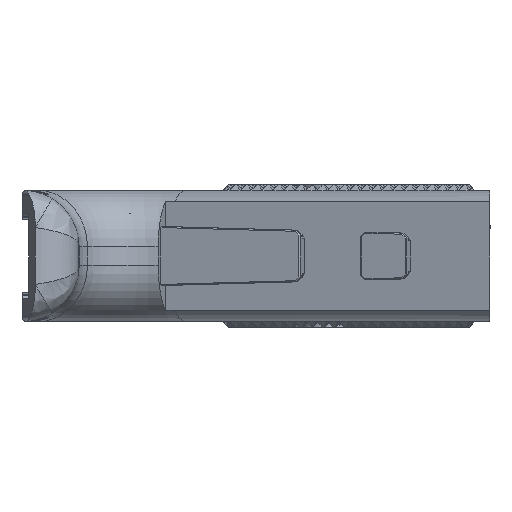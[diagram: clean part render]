
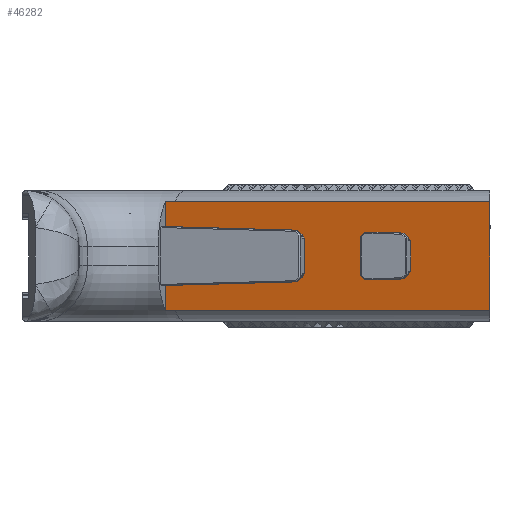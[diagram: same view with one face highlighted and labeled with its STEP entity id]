
A CAD part, left-side view. The second image highlights one B-rep face of the part: STEP entity #46282.
In plain terms, the highlighted planar face has unit normal (-0.951, 0.309, 0).
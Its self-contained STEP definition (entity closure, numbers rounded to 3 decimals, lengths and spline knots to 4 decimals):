
#57=FACE_BOUND('',#19786,.T.);
#5211=LINE('',#88973,#10780);
#5229=LINE('',#89011,#10798);
#5237=LINE('',#89028,#10806);
#5242=LINE('',#89037,#10811);
#5244=LINE('',#89040,#10813);
#5246=LINE('',#89045,#10815);
#5248=LINE('',#89049,#10817);
#5250=LINE('',#89052,#10819);
#5252=LINE('',#89056,#10821);
#5253=LINE('',#89058,#10822);
#5259=LINE('',#89071,#10828);
#5261=LINE('',#89075,#10830);
#5262=LINE('',#89078,#10831);
#5264=LINE('',#89082,#10833);
#5265=LINE('',#89092,#10834);
#5266=LINE('',#89094,#10835);
#5267=LINE('',#89096,#10836);
#5268=LINE('',#89106,#10837);
#5269=LINE('',#89107,#10838);
#10780=VECTOR('',#59780,0.3937);
#10798=VECTOR('',#59816,0.3937);
#10806=VECTOR('',#59830,0.3937);
#10811=VECTOR('',#59839,0.3937);
#10813=VECTOR('',#59843,0.3937);
#10815=VECTOR('',#59847,0.3937);
#10817=VECTOR('',#59851,0.3937);
#10819=VECTOR('',#59855,0.3937);
#10821=VECTOR('',#59859,0.3937);
#10822=VECTOR('',#59862,0.3937);
#10828=VECTOR('',#59878,0.3937);
#10830=VECTOR('',#59882,0.3937);
#10831=VECTOR('',#59885,0.3937);
#10833=VECTOR('',#59889,0.3937);
#10834=VECTOR('',#59890,0.3937);
#10835=VECTOR('',#59891,0.3937);
#10836=VECTOR('',#59892,0.3937);
#10837=VECTOR('',#59893,0.3937);
#10838=VECTOR('',#59894,0.3937);
#13953=PLANE('',#49273);
#16778=FACE_OUTER_BOUND('',#19785,.T.);
#19785=EDGE_LOOP('',(#41315,#41316,#41317,#41318,#41319,#41320,#41321,#41322,
#41323,#41324,#41325,#41326));
#19786=EDGE_LOOP('',(#41327,#41328,#41329,#41330,#41331,#41332,#41333,#41334,
#41335));
#20582=B_SPLINE_CURVE_WITH_KNOTS('',3,(#89084,#89085,#89086,#89087,#89088,
#89089,#89090),.UNSPECIFIED.,.F.,.F.,(4,3,4),(0.,0.1181,0.2155),
 .UNSPECIFIED.);
#20583=B_SPLINE_CURVE_WITH_KNOTS('',3,(#89098,#89099,#89100,#89101,#89102,
#89103,#89104),.UNSPECIFIED.,.F.,.F.,(4,3,4),(-0.2155,-0.1181,
0.),.UNSPECIFIED.);
#23615=VERTEX_POINT('',#88970);
#23616=VERTEX_POINT('',#88972);
#23626=VERTEX_POINT('',#89008);
#23627=VERTEX_POINT('',#89010);
#23632=VERTEX_POINT('',#89025);
#23633=VERTEX_POINT('',#89027);
#23635=VERTEX_POINT('',#89036);
#23636=VERTEX_POINT('',#89042);
#23637=VERTEX_POINT('',#89044);
#23638=VERTEX_POINT('',#89048);
#23639=VERTEX_POINT('',#89054);
#23641=VERTEX_POINT('',#89069);
#23642=VERTEX_POINT('',#89073);
#23643=VERTEX_POINT('',#89077);
#23644=VERTEX_POINT('',#89081);
#23645=VERTEX_POINT('',#89083);
#23646=VERTEX_POINT('',#89091);
#23647=VERTEX_POINT('',#89093);
#23648=VERTEX_POINT('',#89095);
#23649=VERTEX_POINT('',#89097);
#23650=VERTEX_POINT('',#89105);
#29614=EDGE_CURVE('',#23616,#23615,#5211,.T.);
#29632=EDGE_CURVE('',#23626,#23627,#5229,.T.);
#29640=EDGE_CURVE('',#23632,#23633,#5237,.F.);
#29645=EDGE_CURVE('',#23616,#23635,#5242,.F.);
#29647=EDGE_CURVE('',#23632,#23635,#5244,.T.);
#29649=EDGE_CURVE('',#23636,#23637,#5246,.F.);
#29651=EDGE_CURVE('',#23638,#23637,#5248,.T.);
#29653=EDGE_CURVE('',#23636,#23633,#5250,.T.);
#29655=EDGE_CURVE('',#23639,#23615,#5252,.F.);
#29656=EDGE_CURVE('',#23638,#23639,#5253,.F.);
#29662=EDGE_CURVE('',#23641,#23626,#5259,.F.);
#29664=EDGE_CURVE('',#23641,#23642,#5261,.T.);
#29665=EDGE_CURVE('',#23627,#23643,#5262,.F.);
#29667=EDGE_CURVE('',#23644,#23642,#5264,.T.);
#29668=EDGE_CURVE('',#23645,#23644,#20582,.T.);
#29669=EDGE_CURVE('',#23646,#23645,#5265,.T.);
#29670=EDGE_CURVE('',#23647,#23646,#5266,.T.);
#29671=EDGE_CURVE('',#23648,#23647,#5267,.T.);
#29672=EDGE_CURVE('',#23649,#23648,#20583,.T.);
#29673=EDGE_CURVE('',#23650,#23649,#5268,.T.);
#29674=EDGE_CURVE('',#23650,#23643,#5269,.T.);
#41315=ORIENTED_EDGE('',*,*,#29664,.T.);
#41316=ORIENTED_EDGE('',*,*,#29667,.F.);
#41317=ORIENTED_EDGE('',*,*,#29668,.F.);
#41318=ORIENTED_EDGE('',*,*,#29669,.F.);
#41319=ORIENTED_EDGE('',*,*,#29670,.F.);
#41320=ORIENTED_EDGE('',*,*,#29671,.F.);
#41321=ORIENTED_EDGE('',*,*,#29672,.F.);
#41322=ORIENTED_EDGE('',*,*,#29673,.F.);
#41323=ORIENTED_EDGE('',*,*,#29674,.T.);
#41324=ORIENTED_EDGE('',*,*,#29665,.F.);
#41325=ORIENTED_EDGE('',*,*,#29632,.F.);
#41326=ORIENTED_EDGE('',*,*,#29662,.F.);
#41327=ORIENTED_EDGE('',*,*,#29614,.T.);
#41328=ORIENTED_EDGE('',*,*,#29655,.F.);
#41329=ORIENTED_EDGE('',*,*,#29656,.F.);
#41330=ORIENTED_EDGE('',*,*,#29651,.T.);
#41331=ORIENTED_EDGE('',*,*,#29649,.F.);
#41332=ORIENTED_EDGE('',*,*,#29653,.T.);
#41333=ORIENTED_EDGE('',*,*,#29640,.F.);
#41334=ORIENTED_EDGE('',*,*,#29647,.T.);
#41335=ORIENTED_EDGE('',*,*,#29645,.F.);
#46282=ADVANCED_FACE('',(#16778,#57),#13953,.T.);
#49273=AXIS2_PLACEMENT_3D('',#89080,#59887,#59888);
#59780=DIRECTION('',(0.,0.,1.));
#59816=DIRECTION('',(0.,0.,1.));
#59830=DIRECTION('',(0.216,0.664,-0.716));
#59839=DIRECTION('',(0.221,0.681,0.698));
#59843=DIRECTION('',(0.309,0.951,-0.026));
#59847=DIRECTION('',(-0.216,-0.664,-0.716));
#59851=DIRECTION('',(-0.309,-0.951,-0.026));
#59855=DIRECTION('',(0.,0.,-1.));
#59859=DIRECTION('',(-0.12,-0.37,0.921));
#59862=DIRECTION('',(-0.221,-0.681,0.698));
#59878=DIRECTION('',(0.216,0.664,-0.716));
#59882=DIRECTION('',(0.309,0.951,-0.026));
#59885=DIRECTION('',(-0.216,-0.664,-0.716));
#59887=DIRECTION('center_axis',(-0.951,0.309,0.));
#59888=DIRECTION('ref_axis',(0.,0.,
1.));
#59889=DIRECTION('',(0.,0.,1.));
#59890=DIRECTION('',(0.309,0.951,0.));
#59891=DIRECTION('',(0.,0.,-1.));
#59892=DIRECTION('',(-0.309,-0.951,0.));
#59893=DIRECTION('',(0.,0.,1.));
#59894=DIRECTION('',(-0.309,-0.951,-0.026));
#88970=CARTESIAN_POINT('',(-2.8962,-0.8838,-0.6352));
#88972=CARTESIAN_POINT('',(-2.8962,-0.8838,-0.9101));
#88973=CARTESIAN_POINT('',(-2.8962,-0.8838,-0.7677));
#89008=CARTESIAN_POINT('',(-2.7262,-0.3607,-0.9245));
#89010=CARTESIAN_POINT('',(-2.7262,-0.3607,-0.6109));
#89011=CARTESIAN_POINT('',(-2.7262,-0.3607,-0.9154));
#89025=CARTESIAN_POINT('',(-3.0247,-1.2792,-0.909));
#89027=CARTESIAN_POINT('',(-3.0277,-1.2886,-0.8989));
#89028=CARTESIAN_POINT('',(-2.9908,-1.1749,-1.0217));
#89036=CARTESIAN_POINT('',(-2.8992,-0.8932,-0.9197));
#89037=CARTESIAN_POINT('',(-2.8709,-0.806,-0.8303));
#89040=CARTESIAN_POINT('',(-3.0469,-1.3476,-0.9072));
#89042=CARTESIAN_POINT('',(-3.0277,-1.2886,-0.6365));
#89044=CARTESIAN_POINT('',(-3.0247,-1.2792,-0.6264));
#89045=CARTESIAN_POINT('',(-2.9908,-1.1749,-0.5138));
#89048=CARTESIAN_POINT('',(-2.8992,-0.8932,-0.6158));
#89049=CARTESIAN_POINT('',(-3.0469,-1.3476,-0.6283));
#89052=CARTESIAN_POINT('',(-3.0277,-1.2886,-0.899));
#89054=CARTESIAN_POINT('',(-2.8984,-0.8905,-0.6185));
#89056=CARTESIAN_POINT('',(-2.885,-0.8493,-0.7213));
#89058=CARTESIAN_POINT('',(-2.8709,-0.806,-0.7051));
#89069=CARTESIAN_POINT('',(-2.7232,-0.3514,-0.9346));
#89071=CARTESIAN_POINT('',(-2.7647,-0.479,-0.7968));
#89073=CARTESIAN_POINT('',(-2.3324,0.8513,-0.9677));
#89075=CARTESIAN_POINT('',(-3.0469,-1.3476,-0.9072));
#89077=CARTESIAN_POINT('',(-2.7232,-0.3514,-0.6008));
#89078=CARTESIAN_POINT('',(-2.7647,-0.479,-0.7386));
#89080=CARTESIAN_POINT('Origin',(-2.8375,-0.7031,-0.7677));
#89081=CARTESIAN_POINT('',(-2.3324,0.8513,-1.2459));
#89082=CARTESIAN_POINT('',(-2.3324,0.8513,-1.0302));
#89083=CARTESIAN_POINT('',(-2.3592,0.7689,-1.2425));
#89084=CARTESIAN_POINT('Ctrl Pts',(-2.3592,0.7689,
-1.2425));
#89085=CARTESIAN_POINT('Ctrl Pts',(-2.3544,0.7836,
-1.2425));
#89086=CARTESIAN_POINT('Ctrl Pts',(-2.3495,0.7986,
-1.2428));
#89087=CARTESIAN_POINT('Ctrl Pts',(-2.3446,0.8138,
-1.2435));
#89088=CARTESIAN_POINT('Ctrl Pts',(-2.3405,0.8264,
-1.2441));
#89089=CARTESIAN_POINT('Ctrl Pts',(-2.3365,0.8388,
-1.2449));
#89090=CARTESIAN_POINT('Ctrl Pts',(-2.3324,0.8513,-1.2459));
#89091=CARTESIAN_POINT('',(-3.2516,-1.9775,-1.2425));
#89092=CARTESIAN_POINT('',(-2.1969,1.2684,-1.2425));
#89093=CARTESIAN_POINT('',(-3.2516,-1.9775,-0.2929));
#89094=CARTESIAN_POINT('',(-3.2516,-1.9775,-0.3839));
#89095=CARTESIAN_POINT('',(-2.3592,0.7689,-0.2929));
#89096=CARTESIAN_POINT('',(-2.6906,-0.2509,-0.2929));
#89097=CARTESIAN_POINT('',(-2.3324,0.8513,-0.2895));
#89098=CARTESIAN_POINT('Ctrl Pts',(-2.3324,0.8513,-0.2895));
#89099=CARTESIAN_POINT('Ctrl Pts',(-2.3365,0.8388,
-0.2905));
#89100=CARTESIAN_POINT('Ctrl Pts',(-2.3405,0.8264,
-0.2913));
#89101=CARTESIAN_POINT('Ctrl Pts',(-2.3446,0.8138,
-0.2919));
#89102=CARTESIAN_POINT('Ctrl Pts',(-2.3495,0.7986,
-0.2926));
#89103=CARTESIAN_POINT('Ctrl Pts',(-2.3544,0.7836,
-0.2929));
#89104=CARTESIAN_POINT('Ctrl Pts',(-2.3592,0.7689,
-0.2929));
#89105=CARTESIAN_POINT('',(-2.3324,0.8513,-0.5677));
#89106=CARTESIAN_POINT('',(-2.3324,0.8513,-0.7677));
#89107=CARTESIAN_POINT('',(-3.0469,-1.3476,-0.6283));
